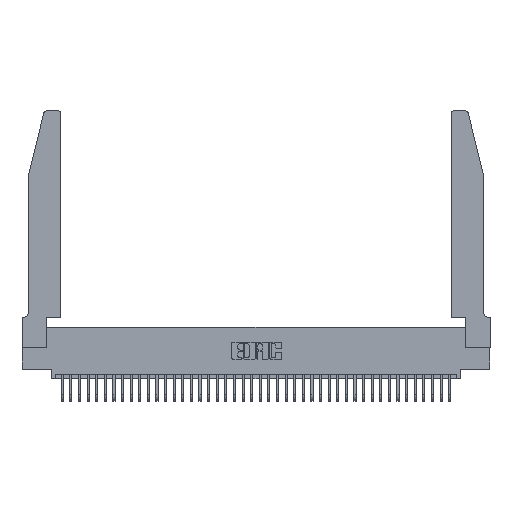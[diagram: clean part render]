
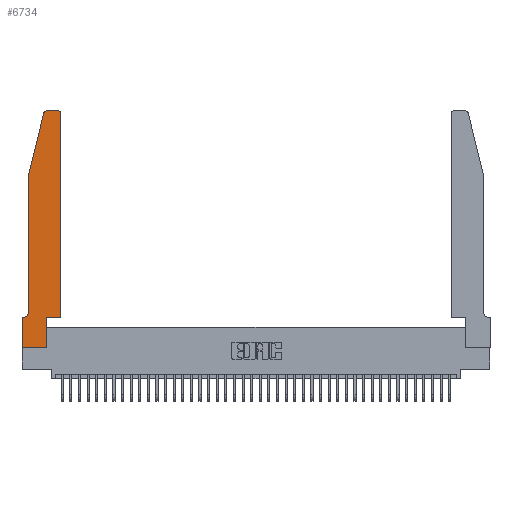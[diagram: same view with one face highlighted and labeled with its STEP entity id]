
A CAD part, top view. The second image highlights one B-rep face of the part: STEP entity #6734.
In plain terms, the highlighted planar face has unit normal (0, 0, 1).
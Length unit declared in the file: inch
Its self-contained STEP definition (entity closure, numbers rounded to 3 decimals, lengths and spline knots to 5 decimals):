
#42 = CARTESIAN_POINT ( 'NONE',  ( 0.0055, 0.42, 0.37 ) ) ;
#332 = ORIENTED_EDGE ( 'NONE', *, *, #33522, .T. ) ;
#614 = CARTESIAN_POINT ( 'NONE',  ( 0., 0.35, 0.37 ) ) ;
#740 = CARTESIAN_POINT ( 'NONE',  ( 0., 0., 0.37 ) ) ;
#1598 = LINE ( 'NONE', #22868, #35146 ) ;
#1822 = ORIENTED_EDGE ( 'NONE', *, *, #11255, .T. ) ;
#2249 = LINE ( 'NONE', #3567, #19485 ) ;
#2755 = LINE ( 'NONE', #5158, #27162 ) ;
#3118 = ORIENTED_EDGE ( 'NONE', *, *, #34856, .T. ) ;
#3567 = CARTESIAN_POINT ( 'NONE',  ( 0.2605, 2.75, 0.37 ) ) ;
#4724 = ORIENTED_EDGE ( 'NONE', *, *, #25962, .T. ) ;
#4896 = CARTESIAN_POINT ( 'NONE',  ( 0.4505, 0.35, 0.37 ) ) ;
#5158 = CARTESIAN_POINT ( 'NONE',  ( 0., 0., 0.37 ) ) ;
#6008 = VECTOR ( 'NONE', #29152, 39.37008 ) ;
#6034 = CARTESIAN_POINT ( 'NONE',  ( 0.4505, 0.35, 0.37 ) ) ;
#6126 = DIRECTION ( 'NONE',  ( 0., 1., 0. ) ) ;
#6321 = CARTESIAN_POINT ( 'NONE',  ( 0.25487, 2.72718, 0.37 ) ) ;
#6590 = AXIS2_PLACEMENT_3D ( 'NONE', #23790, #40003, #10603 ) ;
#6734 = ADVANCED_FACE ( 'NONE', ( #24249 ), #21451, .T. ) ;
#7163 = VERTEX_POINT ( 'NONE', #6321 ) ;
#7191 = DIRECTION ( 'NONE',  ( 0., -1., 0. ) ) ;
#7292 = VERTEX_POINT ( 'NONE', #4896 ) ;
#7398 = CARTESIAN_POINT ( 'NONE',  ( 0.0055, 0.35, 0.37 ) ) ;
#7545 = AXIS2_PLACEMENT_3D ( 'NONE', #22504, #28916, #12482 ) ;
#8139 = CARTESIAN_POINT ( 'NONE',  ( 0.0755, 0.42, 0.37 ) ) ;
#8305 = LINE ( 'NONE', #6034, #18006 ) ;
#8469 = DIRECTION ( 'NONE',  ( 0., 0., 1. ) ) ;
#8603 = DIRECTION ( 'NONE',  ( 1., 0., 0. ) ) ;
#8604 = VECTOR ( 'NONE', #28763, 39.37008 ) ;
#9663 = VECTOR ( 'NONE', #6126, 39.37008 ) ;
#9921 = ORIENTED_EDGE ( 'NONE', *, *, #11911, .T. ) ;
#10167 = VECTOR ( 'NONE', #7191, 39.37008 ) ;
#10603 = DIRECTION ( 'NONE',  ( 1., 0., 0. ) ) ;
#11229 = VERTEX_POINT ( 'NONE', #8139 ) ;
#11255 = EDGE_CURVE ( 'NONE', #7163, #13467, #33531, .T. ) ;
#11770 = DIRECTION ( 'NONE',  ( 1., 0., 0. ) ) ;
#11911 = EDGE_CURVE ( 'NONE', #22106, #23630, #23315, .T. ) ;
#12482 = DIRECTION ( 'NONE',  ( 1., 0., 0. ) ) ;
#12522 = DIRECTION ( 'NONE',  ( 0., 1., 0. ) ) ;
#12594 = VERTEX_POINT ( 'NONE', #35407 ) ;
#12742 = AXIS2_PLACEMENT_3D ( 'NONE', #24882, #8469, #8603 ) ;
#13467 = VERTEX_POINT ( 'NONE', #16856 ) ;
#13471 = ORIENTED_EDGE ( 'NONE', *, *, #22781, .T. ) ;
#14572 = DIRECTION ( 'NONE',  ( 0., -1., 0. ) ) ;
#14962 = VERTEX_POINT ( 'NONE', #36242 ) ;
#15048 = CIRCLE ( 'NONE', #6590, 0.03 ) ;
#15674 = AXIS2_PLACEMENT_3D ( 'NONE', #42, #39034, #29193 ) ;
#16479 = ORIENTED_EDGE ( 'NONE', *, *, #39187, .T. ) ;
#16856 = CARTESIAN_POINT ( 'NONE',  ( 0.0755, 2., 0.37 ) ) ;
#17445 = EDGE_CURVE ( 'NONE', #36368, #12594, #2755, .T. ) ;
#18006 = VECTOR ( 'NONE', #12522, 39.37008 ) ;
#18064 = CARTESIAN_POINT ( 'NONE',  ( 0.4205, 2.75, 0.37 ) ) ;
#19485 = VECTOR ( 'NONE', #22801, 39.37008 ) ;
#19605 = CARTESIAN_POINT ( 'NONE',  ( 0., 0., 0.37 ) ) ;
#21451 = PLANE ( 'NONE',  #12742 ) ;
#22106 = VERTEX_POINT ( 'NONE', #7398 ) ;
#22504 = CARTESIAN_POINT ( 'NONE',  ( 0.4205, 2.72, 0.37 ) ) ;
#22642 = CIRCLE ( 'NONE', #15674, 0.07 ) ;
#22781 = EDGE_CURVE ( 'NONE', #31745, #7163, #15048, .T. ) ;
#22801 = DIRECTION ( 'NONE',  ( -1., 0., 0. ) ) ;
#22868 = CARTESIAN_POINT ( 'NONE',  ( 0.4505, 0.35, 0.37 ) ) ;
#23315 = LINE ( 'NONE', #25884, #6008 ) ;
#23494 = LINE ( 'NONE', #19605, #10167 ) ;
#23630 = VERTEX_POINT ( 'NONE', #614 ) ;
#23790 = CARTESIAN_POINT ( 'NONE',  ( 0.284, 2.72, 0.37 ) ) ;
#23798 = LINE ( 'NONE', #37420, #39071 ) ;
#24249 = FACE_OUTER_BOUND ( 'NONE', #41726, .T. ) ;
#24369 = CIRCLE ( 'NONE', #7545, 0.03 ) ;
#24882 = CARTESIAN_POINT ( 'NONE',  ( 0., 0.35, 0.37 ) ) ;
#25358 = CARTESIAN_POINT ( 'NONE',  ( 0.2865, 0.35, 0.37 ) ) ;
#25884 = CARTESIAN_POINT ( 'NONE',  ( 0.0755, 0.35, 0.37 ) ) ;
#25962 = EDGE_CURVE ( 'NONE', #33378, #7292, #1598, .T. ) ;
#26641 = ORIENTED_EDGE ( 'NONE', *, *, #17445, .T. ) ;
#26970 = VERTEX_POINT ( 'NONE', #18064 ) ;
#27162 = VECTOR ( 'NONE', #11770, 39.37008 ) ;
#28619 = CARTESIAN_POINT ( 'NONE',  ( 0.0755, 2., 0.37 ) ) ;
#28763 = DIRECTION ( 'NONE',  ( -0.239, -0.971, 0. ) ) ;
#28916 = DIRECTION ( 'NONE',  ( 0., 0., 1. ) ) ;
#29152 = DIRECTION ( 'NONE',  ( -1., 0., 0. ) ) ;
#29193 = DIRECTION ( 'NONE',  ( -1., 0., 0. ) ) ;
#30869 = ORIENTED_EDGE ( 'NONE', *, *, #41595, .T. ) ;
#31693 = EDGE_CURVE ( 'NONE', #23630, #36368, #23494, .T. ) ;
#31745 = VERTEX_POINT ( 'NONE', #33282 ) ;
#32666 = DIRECTION ( 'NONE',  ( 1., 0., 0. ) ) ;
#33282 = CARTESIAN_POINT ( 'NONE',  ( 0.284, 2.75, 0.37 ) ) ;
#33378 = VERTEX_POINT ( 'NONE', #25358 ) ;
#33490 = EDGE_CURVE ( 'NONE', #11229, #22106, #22642, .T. ) ;
#33522 = EDGE_CURVE ( 'NONE', #26970, #31745, #2249, .T. ) ;
#33531 = LINE ( 'NONE', #28619, #8604 ) ;
#33733 = ORIENTED_EDGE ( 'NONE', *, *, #36806, .T. ) ;
#34190 = ORIENTED_EDGE ( 'NONE', *, *, #31693, .T. ) ;
#34856 = EDGE_CURVE ( 'NONE', #12594, #33378, #40831, .T. ) ;
#35146 = VECTOR ( 'NONE', #32666, 39.37008 ) ;
#35407 = CARTESIAN_POINT ( 'NONE',  ( 0.2865, 0., 0.37 ) ) ;
#36242 = CARTESIAN_POINT ( 'NONE',  ( 0.4505, 2.72, 0.37 ) ) ;
#36368 = VERTEX_POINT ( 'NONE', #740 ) ;
#36806 = EDGE_CURVE ( 'NONE', #14962, #26970, #24369, .T. ) ;
#37420 = CARTESIAN_POINT ( 'NONE',  ( 0.0755, 2., 0.37 ) ) ;
#39034 = DIRECTION ( 'NONE',  ( 0., 0., -1. ) ) ;
#39071 = VECTOR ( 'NONE', #14572, 39.37008 ) ;
#39187 = EDGE_CURVE ( 'NONE', #13467, #11229, #23798, .T. ) ;
#39284 = CARTESIAN_POINT ( 'NONE',  ( 0.2865, 0.35, 0.37 ) ) ;
#40003 = DIRECTION ( 'NONE',  ( 0., 0., 1. ) ) ;
#40164 = ORIENTED_EDGE ( 'NONE', *, *, #33490, .T. ) ;
#40831 = LINE ( 'NONE', #39284, #9663 ) ;
#41595 = EDGE_CURVE ( 'NONE', #7292, #14962, #8305, .T. ) ;
#41726 = EDGE_LOOP ( 'NONE', ( #332, #13471, #1822, #16479, #40164, #9921, #34190, #26641, #3118, #4724, #30869, #33733 ) ) ;
